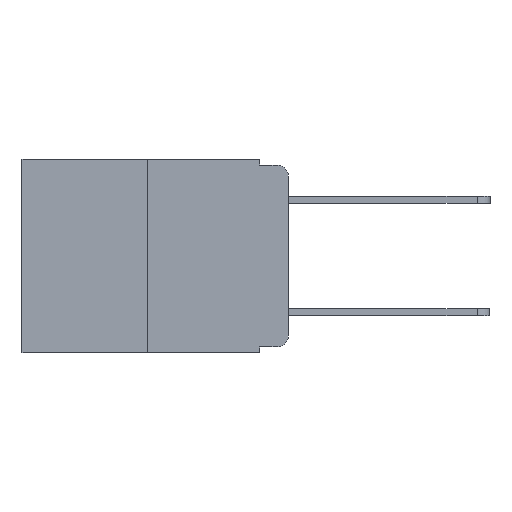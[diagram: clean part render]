
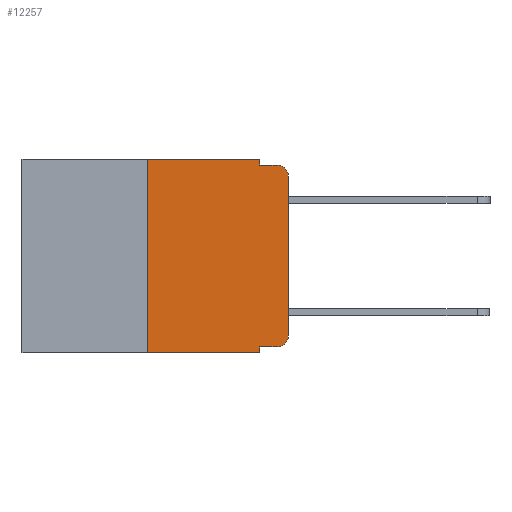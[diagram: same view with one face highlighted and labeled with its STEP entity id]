
A CAD part, left-side view. The second image highlights one B-rep face of the part: STEP entity #12257.
In plain terms, the highlighted planar face has unit normal (-1, 0, 0).
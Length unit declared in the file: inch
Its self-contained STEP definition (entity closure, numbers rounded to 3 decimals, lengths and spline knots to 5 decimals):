
#102 = DIRECTION ( 'NONE',  ( -1., 0., 0. ) ) ;
#117 = CARTESIAN_POINT ( 'NONE',  ( 0., 0.051, -0.01 ) ) ;
#228 = VERTEX_POINT ( 'NONE', #16528 ) ;
#269 = VECTOR ( 'NONE', #3362, 39.37008 ) ;
#363 = VERTEX_POINT ( 'NONE', #4656 ) ;
#517 = VERTEX_POINT ( 'NONE', #3833 ) ;
#704 = VERTEX_POINT ( 'NONE', #117 ) ;
#1259 = ORIENTED_EDGE ( 'NONE', *, *, #3945, .F. ) ;
#1266 = VERTEX_POINT ( 'NONE', #11465 ) ;
#1438 = CARTESIAN_POINT ( 'NONE',  ( 0., 0.473, 0. ) ) ;
#1519 = DIRECTION ( 'NONE',  ( 1., 0., 0. ) ) ;
#1579 = DIRECTION ( 'NONE',  ( 0., -1., 0. ) ) ;
#1667 = DIRECTION ( 'NONE',  ( 0., -1., 0. ) ) ;
#1808 = DIRECTION ( 'NONE',  ( 0., -1., 0. ) ) ;
#1813 = AXIS2_PLACEMENT_3D ( 'NONE', #9823, #102, #11394 ) ;
#2575 = ORIENTED_EDGE ( 'NONE', *, *, #3979, .T. ) ;
#2897 = CARTESIAN_POINT ( 'NONE',  ( 0., 0.051, 0. ) ) ;
#3040 = ORIENTED_EDGE ( 'NONE', *, *, #3913, .F. ) ;
#3153 = EDGE_CURVE ( 'NONE', #1266, #13641, #17200, .T. ) ;
#3362 = DIRECTION ( 'NONE',  ( 0., 0., -1. ) ) ;
#3612 = EDGE_CURVE ( 'NONE', #13439, #517, #14016, .T. ) ;
#3833 = CARTESIAN_POINT ( 'NONE',  ( 0., 0.051, -0.343 ) ) ;
#3882 = EDGE_CURVE ( 'NONE', #11573, #228, #10368, .T. ) ;
#3909 = EDGE_CURVE ( 'NONE', #228, #5569, #9886, .T. ) ;
#3913 = EDGE_CURVE ( 'NONE', #704, #5569, #17365, .T. ) ;
#3945 = EDGE_CURVE ( 'NONE', #13641, #704, #4784, .T. ) ;
#3949 = EDGE_CURVE ( 'NONE', #13439, #1266, #16467, .T. ) ;
#3954 = EDGE_CURVE ( 'NONE', #13454, #517, #4265, .T. ) ;
#3979 = EDGE_CURVE ( 'NONE', #13454, #363, #19412, .T. ) ;
#3982 = EDGE_CURVE ( 'NONE', #363, #11573, #15117, .T. ) ;
#4036 = FACE_OUTER_BOUND ( 'NONE', #19653, .T. ) ;
#4265 = LINE ( 'NONE', #11260, #12065 ) ;
#4656 = CARTESIAN_POINT ( 'NONE',  ( 0., 0.02, -0.333 ) ) ;
#4784 = LINE ( 'NONE', #8007, #269 ) ;
#4798 = CARTESIAN_POINT ( 'NONE',  ( 0., 0., 0. ) ) ;
#5076 = VECTOR ( 'NONE', #8257, 39.37008 ) ;
#5394 = CARTESIAN_POINT ( 'NONE',  ( 0., 0.02, -0.01 ) ) ;
#5569 = VERTEX_POINT ( 'NONE', #5394 ) ;
#5816 = ORIENTED_EDGE ( 'NONE', *, *, #3153, .F. ) ;
#6081 = CARTESIAN_POINT ( 'NONE',  ( 0., 0., -0.313 ) ) ;
#6312 = DIRECTION ( 'NONE',  ( 0., 0., 1. ) ) ;
#6510 = CARTESIAN_POINT ( 'NONE',  ( 0., 0.25, 0. ) ) ;
#6579 = CARTESIAN_POINT ( 'NONE',  ( 0., 0.051, -0.333 ) ) ;
#6674 = CARTESIAN_POINT ( 'NONE',  ( 0., 0.473, 0. ) ) ;
#7927 = CARTESIAN_POINT ( 'NONE',  ( 0., 0.051, -0.01 ) ) ;
#8007 = CARTESIAN_POINT ( 'NONE',  ( 0., 0.051, 0. ) ) ;
#8075 = DIRECTION ( 'NONE',  ( 0., 0., 1. ) ) ;
#8150 = ORIENTED_EDGE ( 'NONE', *, *, #3909, .T. ) ;
#8257 = DIRECTION ( 'NONE',  ( 0., -1., 0. ) ) ;
#8267 = CARTESIAN_POINT ( 'NONE',  ( 0., 0.25, -0.343 ) ) ;
#8422 = VECTOR ( 'NONE', #8075, 39.37008 ) ;
#9068 = ORIENTED_EDGE ( 'NONE', *, *, #3949, .F. ) ;
#9563 = DIRECTION ( 'NONE',  ( -1., 0., 0. ) ) ;
#9796 = CARTESIAN_POINT ( 'NONE',  ( 0., 0.051, -0.333 ) ) ;
#9823 = CARTESIAN_POINT ( 'NONE',  ( 0., 0.02, -0.313 ) ) ;
#9886 = CIRCLE ( 'NONE', #19646, 0.02 ) ;
#10368 = LINE ( 'NONE', #4798, #17826 ) ;
#10386 = VECTOR ( 'NONE', #1667, 39.37008 ) ;
#10527 = ORIENTED_EDGE ( 'NONE', *, *, #3882, .T. ) ;
#11053 = PLANE ( 'NONE',  #18980 ) ;
#11200 = CARTESIAN_POINT ( 'NONE',  ( 0., 0.473, -0.343 ) ) ;
#11260 = CARTESIAN_POINT ( 'NONE',  ( 0., 0.051, 0. ) ) ;
#11394 = DIRECTION ( 'NONE',  ( 0., 0., -1. ) ) ;
#11465 = CARTESIAN_POINT ( 'NONE',  ( 0., 0.25, 0. ) ) ;
#11573 = VERTEX_POINT ( 'NONE', #6081 ) ;
#12065 = VECTOR ( 'NONE', #12810, 39.37008 ) ;
#12257 = ADVANCED_FACE ( 'NONE', ( #4036 ), #11053, .F. ) ;
#12634 = DIRECTION ( 'NONE',  ( 0., 0., -1. ) ) ;
#12810 = DIRECTION ( 'NONE',  ( 0., 0., -1. ) ) ;
#13439 = VERTEX_POINT ( 'NONE', #8267 ) ;
#13454 = VERTEX_POINT ( 'NONE', #9796 ) ;
#13546 = VECTOR ( 'NONE', #1579, 39.37008 ) ;
#13627 = ORIENTED_EDGE ( 'NONE', *, *, #3982, .T. ) ;
#13641 = VERTEX_POINT ( 'NONE', #2897 ) ;
#14016 = LINE ( 'NONE', #11200, #10386 ) ;
#15117 = CIRCLE ( 'NONE', #1813, 0.02 ) ;
#16467 = LINE ( 'NONE', #6510, #8422 ) ;
#16528 = CARTESIAN_POINT ( 'NONE',  ( 0., 0., -0.03 ) ) ;
#17200 = LINE ( 'NONE', #6674, #5076 ) ;
#17289 = ORIENTED_EDGE ( 'NONE', *, *, #3954, .F. ) ;
#17365 = LINE ( 'NONE', #7927, #13546 ) ;
#17826 = VECTOR ( 'NONE', #6312, 39.37008 ) ;
#18500 = CARTESIAN_POINT ( 'NONE',  ( 0., 0.02, -0.03 ) ) ;
#18951 = VECTOR ( 'NONE', #1808, 39.37008 ) ;
#18980 = AXIS2_PLACEMENT_3D ( 'NONE', #1438, #1519, #12634 ) ;
#19412 = LINE ( 'NONE', #6579, #18951 ) ;
#19646 = AXIS2_PLACEMENT_3D ( 'NONE', #18500, #9563, #19940 ) ;
#19653 = EDGE_LOOP ( 'NONE', ( #10527, #8150, #3040, #1259, #5816, #9068, #19912, #17289, #2575, #13627 ) ) ;
#19912 = ORIENTED_EDGE ( 'NONE', *, *, #3612, .T. ) ;
#19940 = DIRECTION ( 'NONE',  ( 0., 0., -1. ) ) ;
